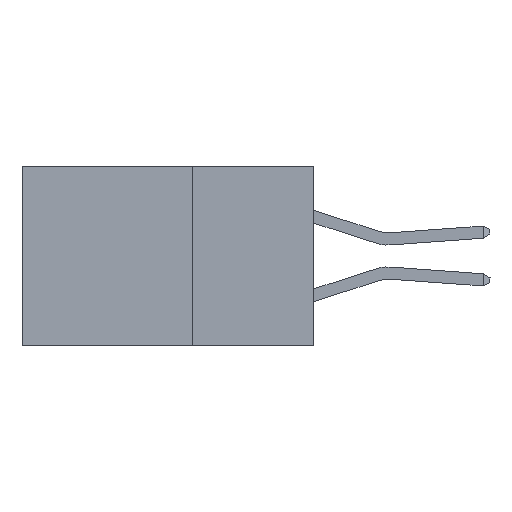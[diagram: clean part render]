
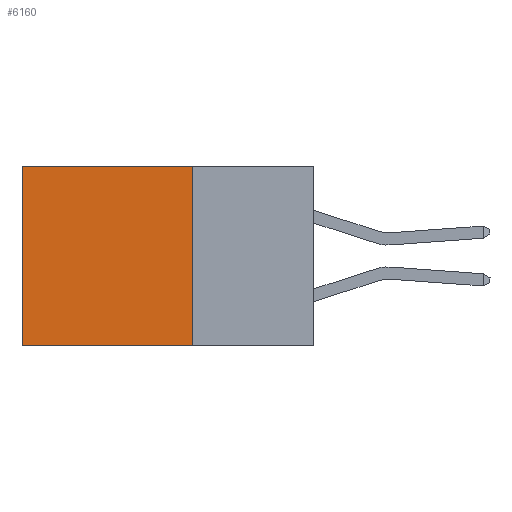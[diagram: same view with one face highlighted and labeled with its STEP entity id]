
A CAD part, left-side view. The second image highlights one B-rep face of the part: STEP entity #6160.
In plain terms, the highlighted planar face has unit normal (-1, 0, 0).
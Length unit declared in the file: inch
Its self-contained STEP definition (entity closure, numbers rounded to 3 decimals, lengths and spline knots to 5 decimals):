
#198 = LINE ( 'NONE', #9036, #5763 ) ;
#1790 = EDGE_CURVE ( 'NONE', #8379, #8296, #198, .T. ) ;
#2770 = CARTESIAN_POINT ( 'NONE',  ( 0.2875, 0.25, -0.37 ) ) ;
#3746 = CARTESIAN_POINT ( 'NONE',  ( 0.2875, 0.6, -0.37 ) ) ;
#4022 = ORIENTED_EDGE ( 'NONE', *, *, #6629, .F. ) ;
#4388 = PLANE ( 'NONE',  #9429 ) ;
#4973 = CARTESIAN_POINT ( 'NONE',  ( 0.2875, 0.25, -0.37 ) ) ;
#5038 = VECTOR ( 'NONE', #14563, 39.37008 ) ;
#5366 = LINE ( 'NONE', #7944, #13975 ) ;
#5698 = DIRECTION ( 'NONE',  ( 0., 0., -1. ) ) ;
#5763 = VECTOR ( 'NONE', #9186, 39.37008 ) ;
#6160 = ADVANCED_FACE ( 'NONE', ( #12640 ), #4388, .F. ) ;
#6469 = CARTESIAN_POINT ( 'NONE',  ( 0.2875, 0.25, 0. ) ) ;
#6629 = EDGE_CURVE ( 'NONE', #12451, #13069, #14764, .T. ) ;
#6676 = CARTESIAN_POINT ( 'NONE',  ( 0.2875, 0.6, 0. ) ) ;
#7519 = EDGE_CURVE ( 'NONE', #8296, #13069, #11052, .T. ) ;
#7850 = DIRECTION ( 'NONE',  ( 0., 0., -1. ) ) ;
#7944 = CARTESIAN_POINT ( 'NONE',  ( 0.2875, 0.25, 0. ) ) ;
#8296 = VERTEX_POINT ( 'NONE', #9710 ) ;
#8379 = VERTEX_POINT ( 'NONE', #6469 ) ;
#8542 = DIRECTION ( 'NONE',  ( 0., 1., 0. ) ) ;
#8941 = CARTESIAN_POINT ( 'NONE',  ( 0.2875, 0.25, 0. ) ) ;
#9036 = CARTESIAN_POINT ( 'NONE',  ( 0.2875, 0.25, 0. ) ) ;
#9186 = DIRECTION ( 'NONE',  ( 0., 1., 0. ) ) ;
#9429 = AXIS2_PLACEMENT_3D ( 'NONE', #8941, #14550, #7850 ) ;
#9710 = CARTESIAN_POINT ( 'NONE',  ( 0.2875, 0.6, 0. ) ) ;
#11052 = LINE ( 'NONE', #6676, #5038 ) ;
#11323 = ORIENTED_EDGE ( 'NONE', *, *, #7519, .T. ) ;
#11524 = ORIENTED_EDGE ( 'NONE', *, *, #1790, .T. ) ;
#11589 = ORIENTED_EDGE ( 'NONE', *, *, #12204, .F. ) ;
#12204 = EDGE_CURVE ( 'NONE', #8379, #12451, #5366, .T. ) ;
#12451 = VERTEX_POINT ( 'NONE', #4973 ) ;
#12640 = FACE_OUTER_BOUND ( 'NONE', #14380, .T. ) ;
#13069 = VERTEX_POINT ( 'NONE', #3746 ) ;
#13975 = VECTOR ( 'NONE', #5698, 39.37008 ) ;
#14380 = EDGE_LOOP ( 'NONE', ( #11323, #4022, #11589, #11524 ) ) ;
#14424 = VECTOR ( 'NONE', #8542, 39.37008 ) ;
#14550 = DIRECTION ( 'NONE',  ( 1., 0., 0. ) ) ;
#14563 = DIRECTION ( 'NONE',  ( 0., 0., -1. ) ) ;
#14764 = LINE ( 'NONE', #2770, #14424 ) ;
